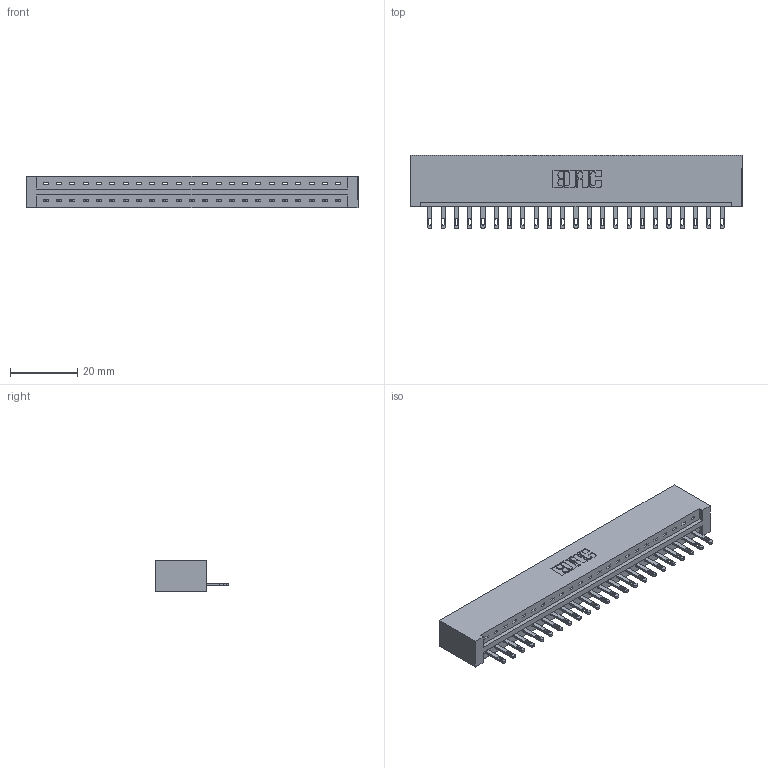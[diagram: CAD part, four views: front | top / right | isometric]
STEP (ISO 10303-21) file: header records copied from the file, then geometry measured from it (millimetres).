
FILE_DESCRIPTION (( 'STEP AP203' ), '1' );
FILE_NAME ('337-023-500-101.STEP', '2019-09-30T14:10:01', ( '' ), ( '' ), 'SwSTEP 2.0', 'SolidWorks 2016', '' );
FILE_SCHEMA (( 'CONFIG_CONTROL_DESIGN' ));
Length unit declared in the file: inch
Products named in the file (3): 345-292-001_345-293-100; 337-023-500-101; 337 Part_No Mounting Lugs
Assembly tree (24 placements, depth 2):
  337-023-500-101
    337 Part_No Mounting Lugs
    345-292-001_345-293-100  x23
Bounding box: 99.01 x 21.85 x 9.4 mm (x, y, z)
Volume: 10805.5 mm3; surface area: 11095.6 mm2
Topology: 24 solids, 24 shells, 1440 faces, 4427 edges, 2950 vertices
Faces by surface type: plane 986, cylinder 454
Entity records: 19207 total; most frequent: CARTESIAN_POINT 3351, ORIENTED_EDGE 3310, DIRECTION 2853, EDGE_CURVE 1655, VECTOR 1531, LINE 1531, VERTEX_POINT 1102, AXIS2_PLACEMENT_3D 661
